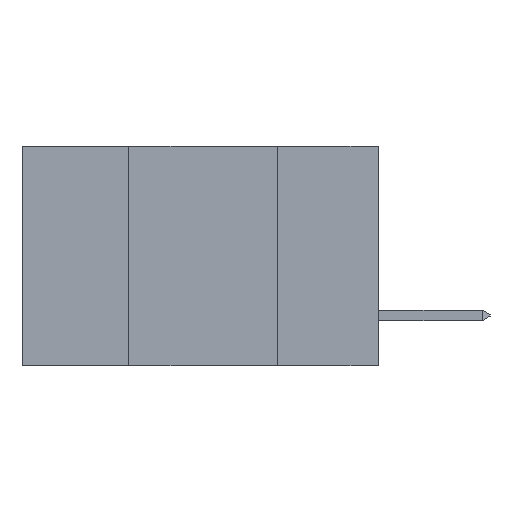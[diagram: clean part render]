
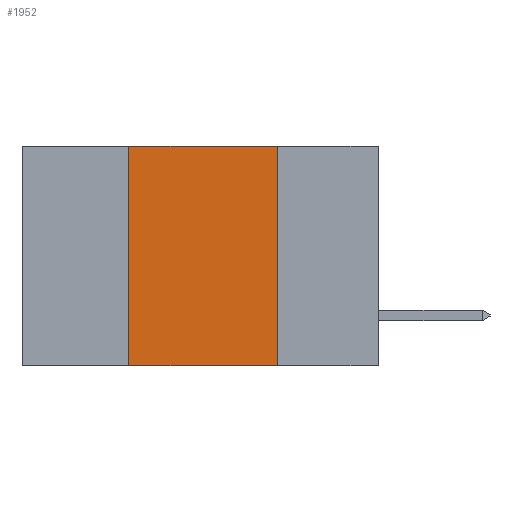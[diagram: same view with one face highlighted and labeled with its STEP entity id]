
A CAD part, left-side view. The second image highlights one B-rep face of the part: STEP entity #1952.
In plain terms, the highlighted planar face has unit normal (-1, 0, 0).
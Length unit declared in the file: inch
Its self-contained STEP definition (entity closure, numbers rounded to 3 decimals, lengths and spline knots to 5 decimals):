
#322 = VERTEX_POINT ( 'NONE', #10366 ) ;
#576 = VECTOR ( 'NONE', #6983, 39.37008 ) ;
#689 = VERTEX_POINT ( 'NONE', #14770 ) ;
#838 = DIRECTION ( 'NONE',  ( 0., 0., -1. ) ) ;
#846 = EDGE_CURVE ( 'NONE', #8957, #689, #5513, .T. ) ;
#1634 = EDGE_LOOP ( 'NONE', ( #8528, #9627, #4235, #4634 ) ) ;
#1952 = ADVANCED_FACE ( 'NONE', ( #8096 ), #8118, .F. ) ;
#2042 = CARTESIAN_POINT ( 'NONE',  ( 0., 0.42, -0.37 ) ) ;
#2471 = VECTOR ( 'NONE', #10520, 39.37008 ) ;
#2739 = CARTESIAN_POINT ( 'NONE',  ( 0., 0.6, 0. ) ) ;
#2745 = EDGE_CURVE ( 'NONE', #689, #322, #14215, .T. ) ;
#4235 = ORIENTED_EDGE ( 'NONE', *, *, #6041, .F. ) ;
#4634 = ORIENTED_EDGE ( 'NONE', *, *, #9642, .T. ) ;
#5357 = VERTEX_POINT ( 'NONE', #2042 ) ;
#5492 = DIRECTION ( 'NONE',  ( 0., -1., 0. ) ) ;
#5513 = LINE ( 'NONE', #2739, #11458 ) ;
#6041 = EDGE_CURVE ( 'NONE', #5357, #8957, #13381, .T. ) ;
#6582 = CARTESIAN_POINT ( 'NONE',  ( 0., 0.42, 0. ) ) ;
#6983 = DIRECTION ( 'NONE',  ( 0., 0., 1. ) ) ;
#7249 = CARTESIAN_POINT ( 'NONE',  ( 0., 0.17, 0. ) ) ;
#8070 = VECTOR ( 'NONE', #838, 39.37008 ) ;
#8096 = FACE_OUTER_BOUND ( 'NONE', #1634, .T. ) ;
#8118 = PLANE ( 'NONE',  #13323 ) ;
#8139 = CARTESIAN_POINT ( 'NONE',  ( 0., 0.42, 0. ) ) ;
#8528 = ORIENTED_EDGE ( 'NONE', *, *, #2745, .F. ) ;
#8957 = VERTEX_POINT ( 'NONE', #8139 ) ;
#9366 = CARTESIAN_POINT ( 'NONE',  ( 0., 0.6, -0.37 ) ) ;
#9627 = ORIENTED_EDGE ( 'NONE', *, *, #846, .F. ) ;
#9642 = EDGE_CURVE ( 'NONE', #5357, #322, #11664, .T. ) ;
#10282 = DIRECTION ( 'NONE',  ( 0., 0., -1. ) ) ;
#10321 = DIRECTION ( 'NONE',  ( 1., 0., 0. ) ) ;
#10366 = CARTESIAN_POINT ( 'NONE',  ( 0., 0.17, -0.37 ) ) ;
#10520 = DIRECTION ( 'NONE',  ( 0., -1., 0. ) ) ;
#11458 = VECTOR ( 'NONE', #5492, 39.37008 ) ;
#11664 = LINE ( 'NONE', #9366, #2471 ) ;
#13323 = AXIS2_PLACEMENT_3D ( 'NONE', #13372, #10321, #10282 ) ;
#13372 = CARTESIAN_POINT ( 'NONE',  ( 0., 0.6, 0. ) ) ;
#13381 = LINE ( 'NONE', #6582, #576 ) ;
#14215 = LINE ( 'NONE', #7249, #8070 ) ;
#14770 = CARTESIAN_POINT ( 'NONE',  ( 0., 0.17, 0. ) ) ;
